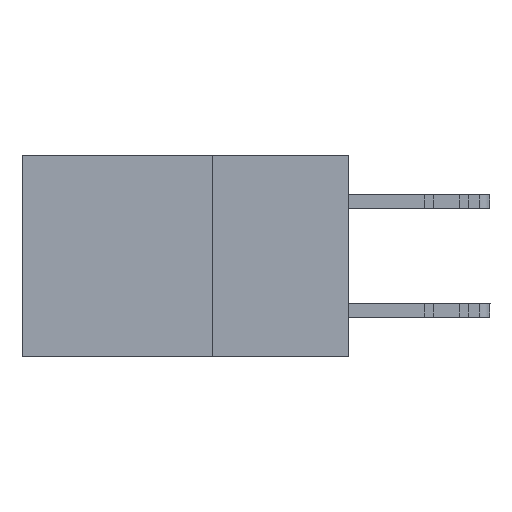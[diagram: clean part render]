
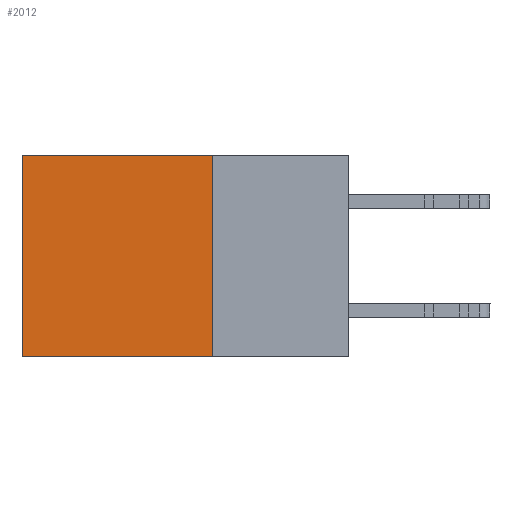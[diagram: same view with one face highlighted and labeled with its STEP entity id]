
A CAD part, left-side view. The second image highlights one B-rep face of the part: STEP entity #2012.
In plain terms, the highlighted planar face has unit normal (-1, 0, 0).
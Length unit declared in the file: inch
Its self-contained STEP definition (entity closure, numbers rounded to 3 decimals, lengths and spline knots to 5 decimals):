
#165 = VECTOR ( 'NONE', #7999, 39.37008 ) ;
#677 = CARTESIAN_POINT ( 'NONE',  ( 0.2615, 0.6, 0. ) ) ;
#1360 = LINE ( 'NONE', #15416, #165 ) ;
#1361 = CARTESIAN_POINT ( 'NONE',  ( 0.2615, 0.6, -0.37 ) ) ;
#1549 = VECTOR ( 'NONE', #11620, 39.37008 ) ;
#1695 = VERTEX_POINT ( 'NONE', #6281 ) ;
#2012 = ADVANCED_FACE ( 'NONE', ( #5534 ), #14768, .F. ) ;
#3291 = EDGE_CURVE ( 'NONE', #20374, #6435, #21576, .T. ) ;
#3317 = DIRECTION ( 'NONE',  ( 0., 0., -1. ) ) ;
#3340 = ORIENTED_EDGE ( 'NONE', *, *, #17571, .F. ) ;
#5095 = CARTESIAN_POINT ( 'NONE',  ( 0.2615, 0.25, -0.37 ) ) ;
#5534 = FACE_OUTER_BOUND ( 'NONE', #18706, .T. ) ;
#6281 = CARTESIAN_POINT ( 'NONE',  ( 0.2615, 0.6, -0.37 ) ) ;
#6435 = VERTEX_POINT ( 'NONE', #22167 ) ;
#7075 = DIRECTION ( 'NONE',  ( 0., 1., 0. ) ) ;
#7768 = ORIENTED_EDGE ( 'NONE', *, *, #3291, .F. ) ;
#7999 = DIRECTION ( 'NONE',  ( 0., 1., 0. ) ) ;
#8676 = VECTOR ( 'NONE', #3317, 39.37008 ) ;
#9172 = CARTESIAN_POINT ( 'NONE',  ( 0.2615, 0.25, -0.37 ) ) ;
#9441 = CARTESIAN_POINT ( 'NONE',  ( 0.2615, 0.25, 0. ) ) ;
#10334 = AXIS2_PLACEMENT_3D ( 'NONE', #9172, #20439, #18708 ) ;
#11620 = DIRECTION ( 'NONE',  ( 0., 0., -1. ) ) ;
#12027 = ORIENTED_EDGE ( 'NONE', *, *, #23691, .T. ) ;
#12936 = VECTOR ( 'NONE', #7075, 39.37008 ) ;
#14768 = PLANE ( 'NONE',  #10334 ) ;
#15416 = CARTESIAN_POINT ( 'NONE',  ( 0.2615, 0.25, 0. ) ) ;
#15529 = EDGE_CURVE ( 'NONE', #19346, #1695, #18648, .T. ) ;
#17571 = EDGE_CURVE ( 'NONE', #6435, #1695, #17939, .T. ) ;
#17939 = LINE ( 'NONE', #5095, #12936 ) ;
#18648 = LINE ( 'NONE', #1361, #8676 ) ;
#18706 = EDGE_LOOP ( 'NONE', ( #22447, #3340, #7768, #12027 ) ) ;
#18708 = DIRECTION ( 'NONE',  ( 0., 0., -1. ) ) ;
#19346 = VERTEX_POINT ( 'NONE', #677 ) ;
#20374 = VERTEX_POINT ( 'NONE', #9441 ) ;
#20439 = DIRECTION ( 'NONE',  ( 1., 0., 0. ) ) ;
#21576 = LINE ( 'NONE', #23403, #1549 ) ;
#22167 = CARTESIAN_POINT ( 'NONE',  ( 0.2615, 0.25, -0.37 ) ) ;
#22447 = ORIENTED_EDGE ( 'NONE', *, *, #15529, .T. ) ;
#23403 = CARTESIAN_POINT ( 'NONE',  ( 0.2615, 0.25, -0.37 ) ) ;
#23691 = EDGE_CURVE ( 'NONE', #20374, #19346, #1360, .T. ) ;
